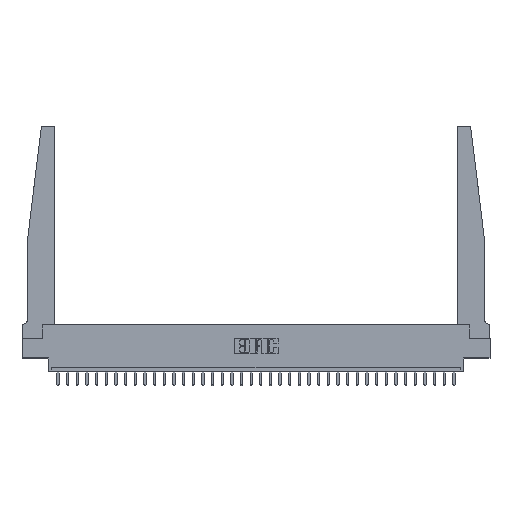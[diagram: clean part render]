
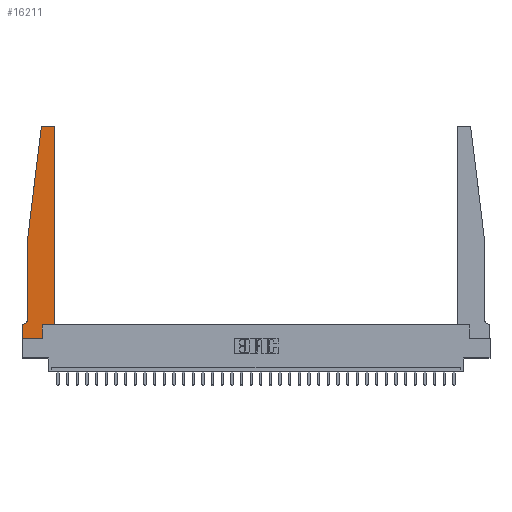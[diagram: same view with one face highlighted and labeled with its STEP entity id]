
A CAD part, top view. The second image highlights one B-rep face of the part: STEP entity #16211.
In plain terms, the highlighted planar face has unit normal (0, 0, 1).
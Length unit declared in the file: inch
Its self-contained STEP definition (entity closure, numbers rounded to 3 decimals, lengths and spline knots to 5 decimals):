
#605 = ORIENTED_EDGE ( 'NONE', *, *, #5984, .T. ) ;
#691 = VERTEX_POINT ( 'NONE', #30858 ) ;
#716 = CARTESIAN_POINT ( 'NONE',  ( 0.065, 1.25, 0.37 ) ) ;
#1235 = VECTOR ( 'NONE', #8430, 39.37008 ) ;
#1384 = EDGE_CURVE ( 'NONE', #12171, #15470, #30077, .T. ) ;
#1400 = VERTEX_POINT ( 'NONE', #4036 ) ;
#1744 = VERTEX_POINT ( 'NONE', #12064 ) ;
#1813 = VECTOR ( 'NONE', #11630, 39.37008 ) ;
#2468 = AXIS2_PLACEMENT_3D ( 'NONE', #22711, #3881, #25232 ) ;
#2695 = VERTEX_POINT ( 'NONE', #13740 ) ;
#3369 = CARTESIAN_POINT ( 'NONE',  ( 0.25, 2.75, 0.37 ) ) ;
#3493 = EDGE_CURVE ( 'NONE', #24841, #1744, #26158, .T. ) ;
#3652 = CARTESIAN_POINT ( 'NONE',  ( 0.24675, 2.72367, 0.37 ) ) ;
#3881 = DIRECTION ( 'NONE',  ( 0., 0., 1. ) ) ;
#4036 = CARTESIAN_POINT ( 'NONE',  ( 0.015, 0.1875, 0.37 ) ) ;
#4542 = DIRECTION ( 'NONE',  ( 0., 0., -1. ) ) ;
#4813 = EDGE_LOOP ( 'NONE', ( #13585, #7382, #25353, #22804, #6619, #9569, #22948, #22411, #26498, #605, #6319, #27888 ) ) ;
#4855 = CARTESIAN_POINT ( 'NONE',  ( 0.015, 0.2375, 0.37 ) ) ;
#5481 = CARTESIAN_POINT ( 'NONE',  ( 0.425, 0.18, 0.37 ) ) ;
#5984 = EDGE_CURVE ( 'NONE', #15470, #2695, #8610, .T. ) ;
#6284 = DIRECTION ( 'NONE',  ( 1., 0., 0. ) ) ;
#6319 = ORIENTED_EDGE ( 'NONE', *, *, #18296, .T. ) ;
#6497 = CARTESIAN_POINT ( 'NONE',  ( 0.395, 2.72, 0.37 ) ) ;
#6523 = CARTESIAN_POINT ( 'NONE',  ( 0.2605, 0.18, 0.37 ) ) ;
#6619 = ORIENTED_EDGE ( 'NONE', *, *, #15961, .T. ) ;
#6967 = DIRECTION ( 'NONE',  ( 0., 0., 1. ) ) ;
#7382 = ORIENTED_EDGE ( 'NONE', *, *, #17682, .T. ) ;
#7658 = DIRECTION ( 'NONE',  ( -0.122, -0.992, 0. ) ) ;
#7808 = DIRECTION ( 'NONE',  ( 0., -1., 0. ) ) ;
#8430 = DIRECTION ( 'NONE',  ( 1., 0., 0. ) ) ;
#8555 = LINE ( 'NONE', #28459, #1813 ) ;
#8610 = LINE ( 'NONE', #5481, #23609 ) ;
#8830 = DIRECTION ( 'NONE',  ( -1., 0., 0. ) ) ;
#9569 = ORIENTED_EDGE ( 'NONE', *, *, #11610, .T. ) ;
#10106 = EDGE_CURVE ( 'NONE', #22292, #18676, #26028, .T. ) ;
#10570 = CIRCLE ( 'NONE', #16904, 0.05 ) ;
#10752 = AXIS2_PLACEMENT_3D ( 'NONE', #6497, #23245, #6284 ) ;
#11104 = VECTOR ( 'NONE', #7808, 39.37008 ) ;
#11322 = DIRECTION ( 'NONE',  ( 0., 1., 0. ) ) ;
#11610 = EDGE_CURVE ( 'NONE', #1400, #22292, #8555, .T. ) ;
#11630 = DIRECTION ( 'NONE',  ( -1., 0., 0. ) ) ;
#12064 = CARTESIAN_POINT ( 'NONE',  ( 0.27653, 2.75, 0.37 ) ) ;
#12171 = VERTEX_POINT ( 'NONE', #23675 ) ;
#13230 = LINE ( 'NONE', #17796, #1235 ) ;
#13585 = ORIENTED_EDGE ( 'NONE', *, *, #3493, .T. ) ;
#13740 = CARTESIAN_POINT ( 'NONE',  ( 0.425, 0.18, 0.37 ) ) ;
#14111 = AXIS2_PLACEMENT_3D ( 'NONE', #16122, #6967, #28279 ) ;
#15470 = VERTEX_POINT ( 'NONE', #22114 ) ;
#15961 = EDGE_CURVE ( 'NONE', #19474, #1400, #10570, .T. ) ;
#16030 = PLANE ( 'NONE',  #2468 ) ;
#16122 = CARTESIAN_POINT ( 'NONE',  ( 0.27653, 2.72, 0.37 ) ) ;
#16211 = ADVANCED_FACE ( 'NONE', ( #21086 ), #16030, .T. ) ;
#16853 = CARTESIAN_POINT ( 'NONE',  ( 0.395, 2.75, 0.37 ) ) ;
#16904 = AXIS2_PLACEMENT_3D ( 'NONE', #4855, #4542, #19109 ) ;
#17283 = VECTOR ( 'NONE', #11322, 39.37008 ) ;
#17517 = LINE ( 'NONE', #29235, #11104 ) ;
#17682 = EDGE_CURVE ( 'NONE', #1744, #23112, #18631, .T. ) ;
#17796 = CARTESIAN_POINT ( 'NONE',  ( 0., 0., 0.37 ) ) ;
#18296 = EDGE_CURVE ( 'NONE', #2695, #691, #21634, .T. ) ;
#18631 = CIRCLE ( 'NONE', #14111, 0.03 ) ;
#18676 = VERTEX_POINT ( 'NONE', #29952 ) ;
#19080 = EDGE_CURVE ( 'NONE', #23112, #28663, #24934, .T. ) ;
#19109 = DIRECTION ( 'NONE',  ( -1., 0., 0. ) ) ;
#19474 = VERTEX_POINT ( 'NONE', #26036 ) ;
#19811 = CARTESIAN_POINT ( 'NONE',  ( 0.425, 0.18, 0.37 ) ) ;
#20755 = EDGE_CURVE ( 'NONE', #691, #24841, #22926, .T. ) ;
#21086 = FACE_OUTER_BOUND ( 'NONE', #4813, .T. ) ;
#21634 = LINE ( 'NONE', #19811, #23847 ) ;
#21928 = CARTESIAN_POINT ( 'NONE',  ( 0.065, 1.25, 0.37 ) ) ;
#22114 = CARTESIAN_POINT ( 'NONE',  ( 0.2605, 0.18, 0.37 ) ) ;
#22292 = VERTEX_POINT ( 'NONE', #28805 ) ;
#22309 = DIRECTION ( 'NONE',  ( 0., -1., 0. ) ) ;
#22411 = ORIENTED_EDGE ( 'NONE', *, *, #25838, .T. ) ;
#22711 = CARTESIAN_POINT ( 'NONE',  ( 0., 0.1875, 0.37 ) ) ;
#22804 = ORIENTED_EDGE ( 'NONE', *, *, #23983, .T. ) ;
#22926 = CIRCLE ( 'NONE', #10752, 0.03 ) ;
#22948 = ORIENTED_EDGE ( 'NONE', *, *, #10106, .T. ) ;
#23030 = VECTOR ( 'NONE', #22309, 39.37008 ) ;
#23112 = VERTEX_POINT ( 'NONE', #3652 ) ;
#23245 = DIRECTION ( 'NONE',  ( 0., 0., 1. ) ) ;
#23609 = VECTOR ( 'NONE', #24652, 39.37008 ) ;
#23675 = CARTESIAN_POINT ( 'NONE',  ( 0.2605, 0., 0.37 ) ) ;
#23847 = VECTOR ( 'NONE', #24387, 39.37008 ) ;
#23983 = EDGE_CURVE ( 'NONE', #28663, #19474, #17517, .T. ) ;
#24387 = DIRECTION ( 'NONE',  ( 0., 1., 0. ) ) ;
#24652 = DIRECTION ( 'NONE',  ( 1., 0., 0. ) ) ;
#24841 = VERTEX_POINT ( 'NONE', #16853 ) ;
#24934 = LINE ( 'NONE', #21928, #30611 ) ;
#25232 = DIRECTION ( 'NONE',  ( 1., 0., 0. ) ) ;
#25353 = ORIENTED_EDGE ( 'NONE', *, *, #19080, .T. ) ;
#25838 = EDGE_CURVE ( 'NONE', #18676, #12171, #13230, .T. ) ;
#26028 = LINE ( 'NONE', #30002, #23030 ) ;
#26036 = CARTESIAN_POINT ( 'NONE',  ( 0.065, 0.2375, 0.37 ) ) ;
#26158 = LINE ( 'NONE', #3369, #28836 ) ;
#26498 = ORIENTED_EDGE ( 'NONE', *, *, #1384, .T. ) ;
#27888 = ORIENTED_EDGE ( 'NONE', *, *, #20755, .T. ) ;
#28279 = DIRECTION ( 'NONE',  ( 1., 0., 0. ) ) ;
#28459 = CARTESIAN_POINT ( 'NONE',  ( 0.065, 0.1875, 0.37 ) ) ;
#28663 = VERTEX_POINT ( 'NONE', #716 ) ;
#28805 = CARTESIAN_POINT ( 'NONE',  ( 0., 0.1875, 0.37 ) ) ;
#28836 = VECTOR ( 'NONE', #8830, 39.37008 ) ;
#29235 = CARTESIAN_POINT ( 'NONE',  ( 0.065, 1.25, 0.37 ) ) ;
#29952 = CARTESIAN_POINT ( 'NONE',  ( 0., 0., 0.37 ) ) ;
#30002 = CARTESIAN_POINT ( 'NONE',  ( 0., 0., 0.37 ) ) ;
#30077 = LINE ( 'NONE', #6523, #17283 ) ;
#30611 = VECTOR ( 'NONE', #7658, 39.37008 ) ;
#30858 = CARTESIAN_POINT ( 'NONE',  ( 0.425, 2.72, 0.37 ) ) ;
